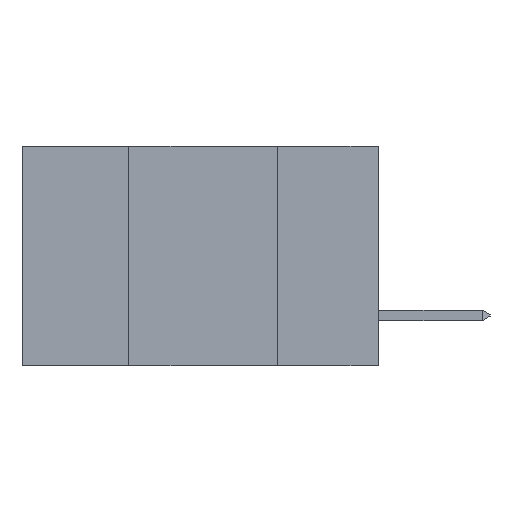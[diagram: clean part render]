
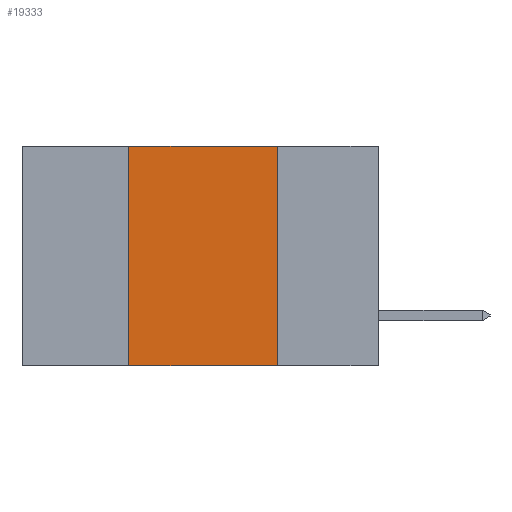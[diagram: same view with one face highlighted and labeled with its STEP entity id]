
A CAD part, left-side view. The second image highlights one B-rep face of the part: STEP entity #19333.
In plain terms, the highlighted planar face has unit normal (-1, 0, 0).
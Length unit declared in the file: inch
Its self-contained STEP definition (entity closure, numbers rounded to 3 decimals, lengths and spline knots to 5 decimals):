
#981 = ORIENTED_EDGE ( 'NONE', *, *, #16360, .T. ) ;
#2406 = VECTOR ( 'NONE', #3553, 39.37008 ) ;
#3039 = VERTEX_POINT ( 'NONE', #16904 ) ;
#3542 = VECTOR ( 'NONE', #4598, 39.37008 ) ;
#3553 = DIRECTION ( 'NONE',  ( 0., -1., 0. ) ) ;
#3921 = EDGE_CURVE ( 'NONE', #19234, #19247, #20947, .T. ) ;
#4564 = LINE ( 'NONE', #15057, #13083 ) ;
#4598 = DIRECTION ( 'NONE',  ( 0., 0., 1. ) ) ;
#4913 = FACE_OUTER_BOUND ( 'NONE', #7962, .T. ) ;
#6085 = CARTESIAN_POINT ( 'NONE',  ( 0., 0.17, 0. ) ) ;
#6101 = ORIENTED_EDGE ( 'NONE', *, *, #11382, .F. ) ;
#7962 = EDGE_LOOP ( 'NONE', ( #9726, #15155, #6101, #981 ) ) ;
#8632 = CARTESIAN_POINT ( 'NONE',  ( 0., 0.6, 0. ) ) ;
#8829 = DIRECTION ( 'NONE',  ( 0., -1., 0. ) ) ;
#9183 = LINE ( 'NONE', #13018, #3542 ) ;
#9726 = ORIENTED_EDGE ( 'NONE', *, *, #12694, .F. ) ;
#9779 = CARTESIAN_POINT ( 'NONE',  ( 0., 0.6, 0. ) ) ;
#11382 = EDGE_CURVE ( 'NONE', #3039, #19234, #9183, .T. ) ;
#11464 = DIRECTION ( 'NONE',  ( 0., 0., -1. ) ) ;
#12694 = EDGE_CURVE ( 'NONE', #19247, #19471, #4564, .T. ) ;
#12724 = AXIS2_PLACEMENT_3D ( 'NONE', #9779, #21485, #11464 ) ;
#13018 = CARTESIAN_POINT ( 'NONE',  ( 0., 0.42, -0.37 ) ) ;
#13083 = VECTOR ( 'NONE', #18466, 39.37008 ) ;
#13537 = CARTESIAN_POINT ( 'NONE',  ( 0., 0.17, -0.37 ) ) ;
#14250 = LINE ( 'NONE', #18944, #18755 ) ;
#15057 = CARTESIAN_POINT ( 'NONE',  ( 0., 0.17, -0.37 ) ) ;
#15155 = ORIENTED_EDGE ( 'NONE', *, *, #3921, .F. ) ;
#16360 = EDGE_CURVE ( 'NONE', #3039, #19471, #14250, .T. ) ;
#16904 = CARTESIAN_POINT ( 'NONE',  ( 0., 0.42, -0.37 ) ) ;
#17931 = CARTESIAN_POINT ( 'NONE',  ( 0., 0.42, 0. ) ) ;
#18466 = DIRECTION ( 'NONE',  ( 0., 0., -1. ) ) ;
#18755 = VECTOR ( 'NONE', #8829, 39.37008 ) ;
#18944 = CARTESIAN_POINT ( 'NONE',  ( 0., 0.6, -0.37 ) ) ;
#19234 = VERTEX_POINT ( 'NONE', #17931 ) ;
#19247 = VERTEX_POINT ( 'NONE', #6085 ) ;
#19333 = ADVANCED_FACE ( 'NONE', ( #4913 ), #21413, .F. ) ;
#19471 = VERTEX_POINT ( 'NONE', #13537 ) ;
#20947 = LINE ( 'NONE', #8632, #2406 ) ;
#21413 = PLANE ( 'NONE',  #12724 ) ;
#21485 = DIRECTION ( 'NONE',  ( 1., 0., 0. ) ) ;
